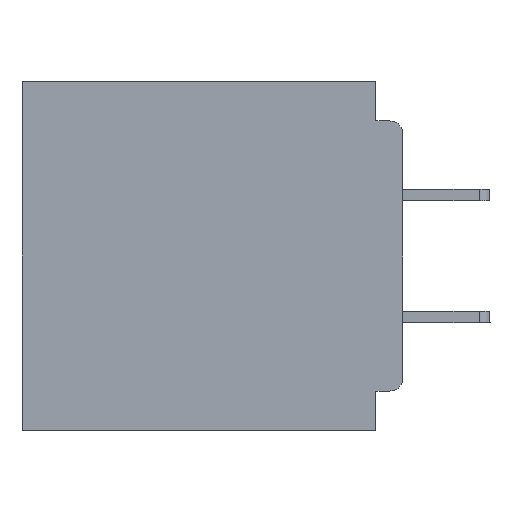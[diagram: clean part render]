
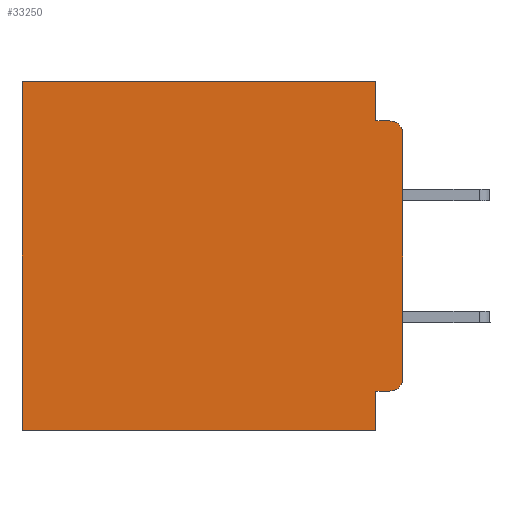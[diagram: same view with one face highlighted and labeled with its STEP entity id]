
A CAD part, left-side view. The second image highlights one B-rep face of the part: STEP entity #33250.
In plain terms, the highlighted planar face has unit normal (-1, 0, 0).
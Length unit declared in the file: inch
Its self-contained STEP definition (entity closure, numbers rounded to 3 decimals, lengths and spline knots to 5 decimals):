
#632 = ORIENTED_EDGE ( 'NONE', *, *, #58563, .F. ) ;
#863 = DIRECTION ( 'NONE',  ( 0., 0., -1. ) ) ;
#1930 = DIRECTION ( 'NONE',  ( 0., 0., -1. ) ) ;
#3123 = VECTOR ( 'NONE', #25322, 39.37008 ) ;
#3339 = EDGE_CURVE ( 'NONE', #37234, #38833, #55838, .T. ) ;
#5581 = VERTEX_POINT ( 'NONE', #33529 ) ;
#5780 = LINE ( 'NONE', #31113, #41260 ) ;
#6677 = EDGE_CURVE ( 'NONE', #38833, #27560, #24594, .T. ) ;
#7881 = VERTEX_POINT ( 'NONE', #41710 ) ;
#10119 = CARTESIAN_POINT ( 'NONE',  ( 0.3, 0.015, -0.34 ) ) ;
#11331 = VECTOR ( 'NONE', #18586, 39.37008 ) ;
#13307 = VECTOR ( 'NONE', #42454, 39.37008 ) ;
#13332 = CARTESIAN_POINT ( 'NONE',  ( 0.3, 0.031, -0.4 ) ) ;
#15021 = DIRECTION ( 'NONE',  ( 0., 0., -1. ) ) ;
#15909 = ORIENTED_EDGE ( 'NONE', *, *, #43765, .F. ) ;
#16507 = EDGE_CURVE ( 'NONE', #5581, #43958, #54127, .T. ) ;
#17821 = CARTESIAN_POINT ( 'NONE',  ( 0.3, 0., -0.4 ) ) ;
#17961 = LINE ( 'NONE', #41502, #54757 ) ;
#18217 = EDGE_CURVE ( 'NONE', #7881, #27560, #17961, .T. ) ;
#18245 = ORIENTED_EDGE ( 'NONE', *, *, #41798, .F. ) ;
#18586 = DIRECTION ( 'NONE',  ( 0., 1., 0. ) ) ;
#18678 = DIRECTION ( 'NONE',  ( 0., -1., 0. ) ) ;
#19690 = ORIENTED_EDGE ( 'NONE', *, *, #37354, .T. ) ;
#20139 = VERTEX_POINT ( 'NONE', #33684 ) ;
#20315 = CARTESIAN_POINT ( 'NONE',  ( 0.3, 0.015, -0.045 ) ) ;
#21540 = VERTEX_POINT ( 'NONE', #20315 ) ;
#23793 = VECTOR ( 'NONE', #46582, 39.37008 ) ;
#24104 = LINE ( 'NONE', #52185, #11331 ) ;
#24594 = LINE ( 'NONE', #37630, #13307 ) ;
#25301 = CARTESIAN_POINT ( 'NONE',  ( 0.3, 0.015, -0.06 ) ) ;
#25322 = DIRECTION ( 'NONE',  ( 0., 0., -1. ) ) ;
#25482 = LINE ( 'NONE', #52261, #60708 ) ;
#27560 = VERTEX_POINT ( 'NONE', #47050 ) ;
#29497 = ORIENTED_EDGE ( 'NONE', *, *, #3339, .F. ) ;
#29511 = CIRCLE ( 'NONE', #50813, 0.015 ) ;
#30101 = DIRECTION ( 'NONE',  ( 0., 0., -1. ) ) ;
#30405 = CARTESIAN_POINT ( 'NONE',  ( 0.3, 0.031, -0.4 ) ) ;
#30439 = AXIS2_PLACEMENT_3D ( 'NONE', #45158, #30871, #1930 ) ;
#30871 = DIRECTION ( 'NONE',  ( 1., 0., 0. ) ) ;
#31113 = CARTESIAN_POINT ( 'NONE',  ( 0.3, 0., 0. ) ) ;
#33121 = EDGE_CURVE ( 'NONE', #20139, #43742, #60705, .T. ) ;
#33185 = CARTESIAN_POINT ( 'NONE',  ( 0.3, 0.031, -0.045 ) ) ;
#33250 = ADVANCED_FACE ( 'NONE', ( #38963 ), #59595, .F. ) ;
#33298 = CARTESIAN_POINT ( 'NONE',  ( 0.3, 0., -0.06 ) ) ;
#33529 = CARTESIAN_POINT ( 'NONE',  ( 0.3, 0.015, -0.355 ) ) ;
#33684 = CARTESIAN_POINT ( 'NONE',  ( 0.3, 0.031, 0. ) ) ;
#33707 = VECTOR ( 'NONE', #863, 39.37008 ) ;
#35097 = LINE ( 'NONE', #17821, #23793 ) ;
#36223 = ORIENTED_EDGE ( 'NONE', *, *, #33121, .F. ) ;
#37234 = VERTEX_POINT ( 'NONE', #39773 ) ;
#37354 = EDGE_CURVE ( 'NONE', #20139, #7881, #5780, .T. ) ;
#37630 = CARTESIAN_POINT ( 'NONE',  ( 0.3, 0., -0.4 ) ) ;
#37768 = ORIENTED_EDGE ( 'NONE', *, *, #6677, .F. ) ;
#38833 = VERTEX_POINT ( 'NONE', #30405 ) ;
#38963 = FACE_OUTER_BOUND ( 'NONE', #58796, .T. ) ;
#38987 = DIRECTION ( 'NONE',  ( 0., 1., 0. ) ) ;
#39773 = CARTESIAN_POINT ( 'NONE',  ( 0.3, 0.031, -0.355 ) ) ;
#40096 = ORIENTED_EDGE ( 'NONE', *, *, #16507, .T. ) ;
#41260 = VECTOR ( 'NONE', #38987, 39.37008 ) ;
#41502 = CARTESIAN_POINT ( 'NONE',  ( 0.3, 0.437, -0.4 ) ) ;
#41710 = CARTESIAN_POINT ( 'NONE',  ( 0.3, 0.437, 0. ) ) ;
#41798 = EDGE_CURVE ( 'NONE', #5581, #37234, #24104, .T. ) ;
#42454 = DIRECTION ( 'NONE',  ( 0., 1., 0. ) ) ;
#43000 = ORIENTED_EDGE ( 'NONE', *, *, #18217, .T. ) ;
#43742 = VERTEX_POINT ( 'NONE', #33185 ) ;
#43765 = EDGE_CURVE ( 'NONE', #43742, #21540, #25482, .T. ) ;
#43775 = DIRECTION ( 'NONE',  ( -1., 0., 0. ) ) ;
#43958 = VERTEX_POINT ( 'NONE', #44289 ) ;
#44289 = CARTESIAN_POINT ( 'NONE',  ( 0.3, 0., -0.34 ) ) ;
#45158 = CARTESIAN_POINT ( 'NONE',  ( 0.3, 0., -0.4 ) ) ;
#45193 = ORIENTED_EDGE ( 'NONE', *, *, #54532, .T. ) ;
#46582 = DIRECTION ( 'NONE',  ( 0., 0., -1. ) ) ;
#47050 = CARTESIAN_POINT ( 'NONE',  ( 0.3, 0.437, -0.4 ) ) ;
#50813 = AXIS2_PLACEMENT_3D ( 'NONE', #25301, #58804, #30101 ) ;
#52185 = CARTESIAN_POINT ( 'NONE',  ( 0.3, 0., -0.355 ) ) ;
#52261 = CARTESIAN_POINT ( 'NONE',  ( 0.3, 0., -0.045 ) ) ;
#54127 = CIRCLE ( 'NONE', #58071, 0.015 ) ;
#54532 = EDGE_CURVE ( 'NONE', #61783, #21540, #29511, .T. ) ;
#54757 = VECTOR ( 'NONE', #55724, 39.37008 ) ;
#55724 = DIRECTION ( 'NONE',  ( 0., 0., -1. ) ) ;
#55838 = LINE ( 'NONE', #13332, #3123 ) ;
#58071 = AXIS2_PLACEMENT_3D ( 'NONE', #10119, #43775, #15021 ) ;
#58544 = CARTESIAN_POINT ( 'NONE',  ( 0.3, 0.031, 0. ) ) ;
#58563 = EDGE_CURVE ( 'NONE', #61783, #43958, #35097, .T. ) ;
#58796 = EDGE_LOOP ( 'NONE', ( #632, #45193, #15909, #36223, #19690, #43000, #37768, #29497, #18245, #40096 ) ) ;
#58804 = DIRECTION ( 'NONE',  ( -1., 0., 0. ) ) ;
#59595 = PLANE ( 'NONE',  #30439 ) ;
#60705 = LINE ( 'NONE', #58544, #33707 ) ;
#60708 = VECTOR ( 'NONE', #18678, 39.37008 ) ;
#61783 = VERTEX_POINT ( 'NONE', #33298 ) ;
